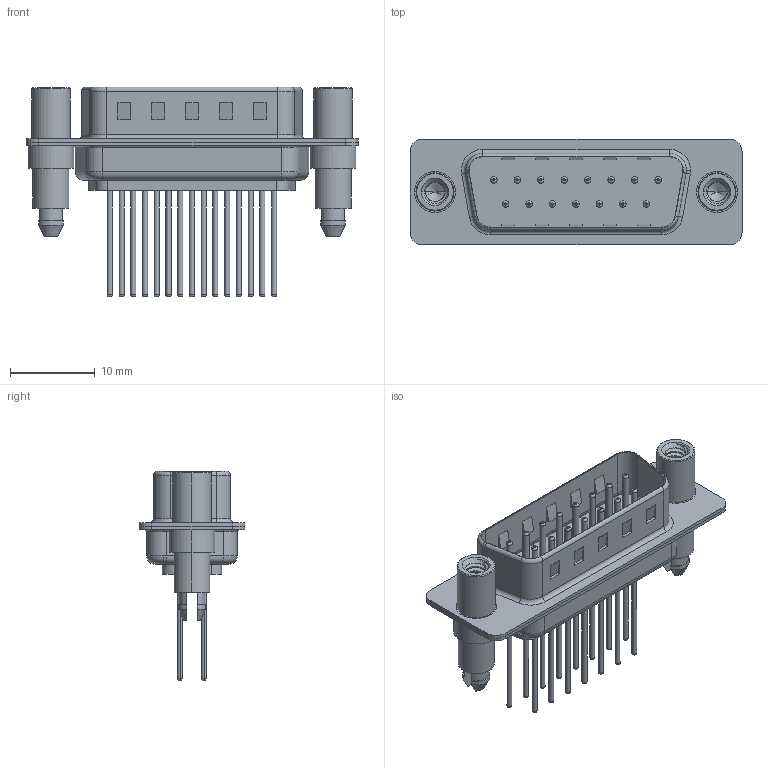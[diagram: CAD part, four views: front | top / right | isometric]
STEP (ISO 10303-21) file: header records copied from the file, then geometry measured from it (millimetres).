
FILE_DESCRIPTION (( 'STEP AP203' ), '1' );
FILE_NAME ('627-M15-223-BT6.STEP', '2020-07-16T23:51:32', ( '' ), ( '' ), 'SwSTEP 2.0', 'SolidWorks 2020', '' );
FILE_SCHEMA (( 'CONFIG_CONTROL_DESIGN' ));
Length unit declared in the file: millimetre
Products named in the file (7): 627M Housing_15 Contacts; 627M 4-40 Threaded Standoff and Boardlock; 627M Contact Row 2_23; 627M Shell Rear_15 Contacts; 627M Shell Front_15 Contacts; 627-M15-223-BT6; 627M Contact Row 1_23
Assembly tree (20 placements, depth 2):
  627-M15-223-BT6
    627M Housing_15 Contacts
    627M Shell Front_15 Contacts
    627M Shell Rear_15 Contacts
    627M Contact Row 1_23  x8
    627M Contact Row 2_23  x7
    627M 4-40 Threaded Standoff and Boardlock  x2
Bounding box: 39.2 x 12.5 x 24.77 mm (x, y, z)
Volume: 2210.9 mm3; surface area: 5470.5 mm2
Topology: 20 solids, 20 shells, 947 faces, 2095 edges, 1280 vertices
Faces by surface type: cylinder 371, torus 290, plane 262, cone 18, bspline 6
Entity records: 17226 total; most frequent: CARTESIAN_POINT 3743, DIRECTION 2791, ORIENTED_EDGE 2440, EDGE_CURVE 1220, AXIS2_PLACEMENT_3D 1104, VERTEX_POINT 771, EDGE_LOOP 623, VECTOR 583
